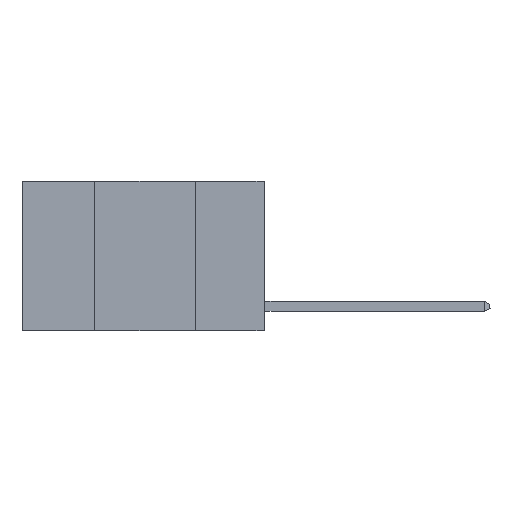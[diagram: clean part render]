
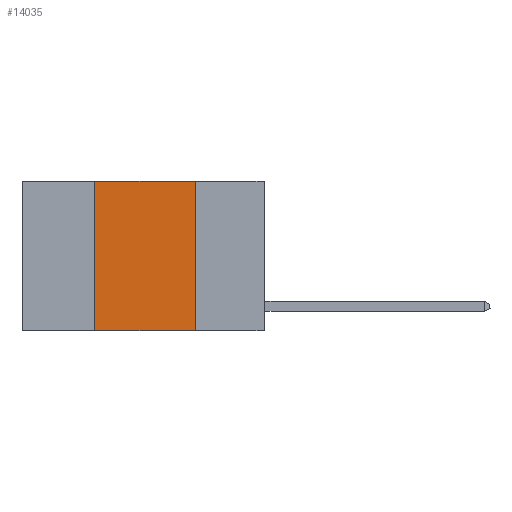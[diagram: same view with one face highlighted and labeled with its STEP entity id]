
A CAD part, left-side view. The second image highlights one B-rep face of the part: STEP entity #14035.
In plain terms, the highlighted planar face has unit normal (-1, 0, 0).
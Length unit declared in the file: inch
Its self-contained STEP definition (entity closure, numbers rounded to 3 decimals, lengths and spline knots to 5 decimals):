
#120 = VECTOR ( 'NONE', #6570, 39.37008 ) ;
#604 = EDGE_CURVE ( 'NONE', #15193, #9259, #9248, .T. ) ;
#1485 = CARTESIAN_POINT ( 'NONE',  ( 0., 0.17, 0. ) ) ;
#3842 = LINE ( 'NONE', #5153, #120 ) ;
#4229 = CARTESIAN_POINT ( 'NONE',  ( 0., 0.17, 0. ) ) ;
#4353 = DIRECTION ( 'NONE',  ( 1., 0., 0. ) ) ;
#4737 = VECTOR ( 'NONE', #8424, 39.37008 ) ;
#5118 = VERTEX_POINT ( 'NONE', #8499 ) ;
#5153 = CARTESIAN_POINT ( 'NONE',  ( 0., 0.6, 0. ) ) ;
#6374 = ORIENTED_EDGE ( 'NONE', *, *, #12679, .F. ) ;
#6570 = DIRECTION ( 'NONE',  ( 0., -1., 0. ) ) ;
#7378 = FACE_OUTER_BOUND ( 'NONE', #8794, .T. ) ;
#7876 = ORIENTED_EDGE ( 'NONE', *, *, #604, .T. ) ;
#8153 = CARTESIAN_POINT ( 'NONE',  ( 0., 0.17, -0.37 ) ) ;
#8268 = CARTESIAN_POINT ( 'NONE',  ( 0., 0.6, -0.37 ) ) ;
#8340 = EDGE_CURVE ( 'NONE', #13356, #9259, #8432, .T. ) ;
#8424 = DIRECTION ( 'NONE',  ( 0., 0., -1. ) ) ;
#8432 = LINE ( 'NONE', #4229, #4737 ) ;
#8499 = CARTESIAN_POINT ( 'NONE',  ( 0., 0.42, 0. ) ) ;
#8794 = EDGE_LOOP ( 'NONE', ( #11167, #15881, #6374, #7876 ) ) ;
#9248 = LINE ( 'NONE', #8268, #15690 ) ;
#9259 = VERTEX_POINT ( 'NONE', #8153 ) ;
#9611 = VECTOR ( 'NONE', #13590, 39.37008 ) ;
#9690 = DIRECTION ( 'NONE',  ( 0., -1., 0. ) ) ;
#11167 = ORIENTED_EDGE ( 'NONE', *, *, #8340, .F. ) ;
#11655 = AXIS2_PLACEMENT_3D ( 'NONE', #12653, #4353, #14034 ) ;
#12218 = CARTESIAN_POINT ( 'NONE',  ( 0., 0.42, 0. ) ) ;
#12653 = CARTESIAN_POINT ( 'NONE',  ( 0., 0.6, 0. ) ) ;
#12679 = EDGE_CURVE ( 'NONE', #15193, #5118, #16927, .T. ) ;
#13356 = VERTEX_POINT ( 'NONE', #1485 ) ;
#13590 = DIRECTION ( 'NONE',  ( 0., 0., 1. ) ) ;
#14034 = DIRECTION ( 'NONE',  ( 0., 0., -1. ) ) ;
#14035 = ADVANCED_FACE ( 'NONE', ( #7378 ), #16760, .F. ) ;
#14795 = EDGE_CURVE ( 'NONE', #5118, #13356, #3842, .T. ) ;
#15193 = VERTEX_POINT ( 'NONE', #15977 ) ;
#15690 = VECTOR ( 'NONE', #9690, 39.37008 ) ;
#15881 = ORIENTED_EDGE ( 'NONE', *, *, #14795, .F. ) ;
#15977 = CARTESIAN_POINT ( 'NONE',  ( 0., 0.42, -0.37 ) ) ;
#16760 = PLANE ( 'NONE',  #11655 ) ;
#16927 = LINE ( 'NONE', #12218, #9611 ) ;
